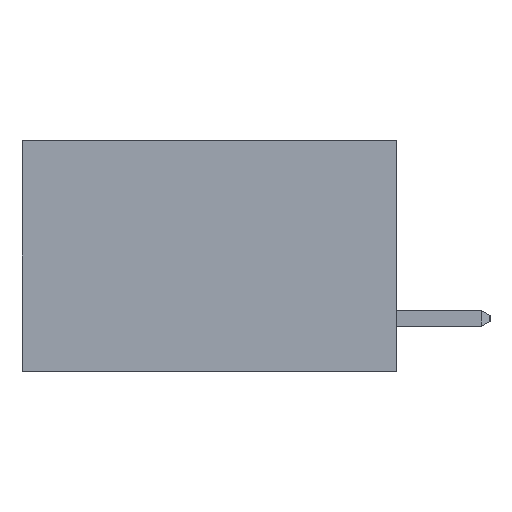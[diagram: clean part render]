
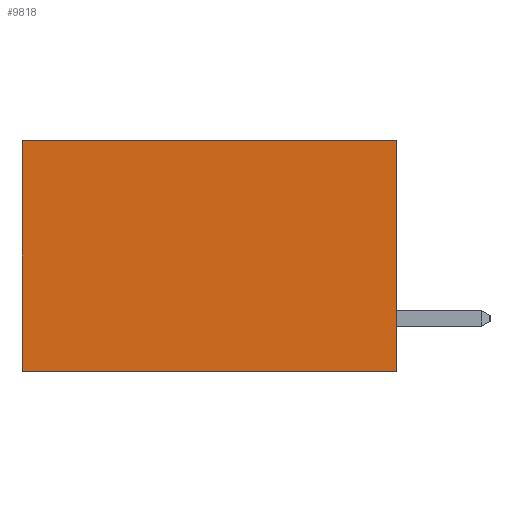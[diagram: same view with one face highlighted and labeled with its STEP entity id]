
A CAD part, left-side view. The second image highlights one B-rep face of the part: STEP entity #9818.
In plain terms, the highlighted planar face has unit normal (-1, 0, 0).
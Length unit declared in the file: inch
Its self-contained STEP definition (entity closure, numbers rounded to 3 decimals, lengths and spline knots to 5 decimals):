
#270 = CARTESIAN_POINT ( 'NONE',  ( 0.298, 0., 0. ) ) ;
#298 = LINE ( 'NONE', #11627, #12478 ) ;
#893 = VERTEX_POINT ( 'NONE', #12988 ) ;
#1684 = VERTEX_POINT ( 'NONE', #5864 ) ;
#2046 = LINE ( 'NONE', #10620, #7878 ) ;
#2406 = EDGE_LOOP ( 'NONE', ( #6444, #13858, #11704, #6688 ) ) ;
#2686 = DIRECTION ( 'NONE',  ( 0., 0., -1. ) ) ;
#3616 = CARTESIAN_POINT ( 'NONE',  ( 0.298, 0., -0.37 ) ) ;
#4255 = VERTEX_POINT ( 'NONE', #12004 ) ;
#4386 = VECTOR ( 'NONE', #2686, 39.37008 ) ;
#4755 = LINE ( 'NONE', #270, #4386 ) ;
#5110 = AXIS2_PLACEMENT_3D ( 'NONE', #6878, #6774, #6847 ) ;
#5672 = VERTEX_POINT ( 'NONE', #10574 ) ;
#5864 = CARTESIAN_POINT ( 'NONE',  ( 0.298, 0.6, 0. ) ) ;
#6444 = ORIENTED_EDGE ( 'NONE', *, *, #7869, .T. ) ;
#6688 = ORIENTED_EDGE ( 'NONE', *, *, #7137, .T. ) ;
#6774 = DIRECTION ( 'NONE',  ( 1., 0., 0. ) ) ;
#6847 = DIRECTION ( 'NONE',  ( 0., 0., -1. ) ) ;
#6878 = CARTESIAN_POINT ( 'NONE',  ( 0.298, 0., 0. ) ) ;
#7002 = PLANE ( 'NONE',  #5110 ) ;
#7032 = DIRECTION ( 'NONE',  ( 0., 1., 0. ) ) ;
#7040 = EDGE_CURVE ( 'NONE', #4255, #5672, #4755, .T. ) ;
#7137 = EDGE_CURVE ( 'NONE', #4255, #1684, #298, .T. ) ;
#7869 = EDGE_CURVE ( 'NONE', #1684, #893, #2046, .T. ) ;
#7878 = VECTOR ( 'NONE', #10051, 39.37008 ) ;
#8053 = EDGE_CURVE ( 'NONE', #5672, #893, #11589, .T. ) ;
#9304 = FACE_OUTER_BOUND ( 'NONE', #2406, .T. ) ;
#9818 = ADVANCED_FACE ( 'NONE', ( #9304 ), #7002, .F. ) ;
#10051 = DIRECTION ( 'NONE',  ( 0., 0., -1. ) ) ;
#10574 = CARTESIAN_POINT ( 'NONE',  ( 0.298, 0., -0.37 ) ) ;
#10620 = CARTESIAN_POINT ( 'NONE',  ( 0.298, 0.6, 0. ) ) ;
#11589 = LINE ( 'NONE', #3616, #12331 ) ;
#11627 = CARTESIAN_POINT ( 'NONE',  ( 0.298, 0., 0. ) ) ;
#11704 = ORIENTED_EDGE ( 'NONE', *, *, #7040, .F. ) ;
#12004 = CARTESIAN_POINT ( 'NONE',  ( 0.298, 0., 0. ) ) ;
#12331 = VECTOR ( 'NONE', #7032, 39.37008 ) ;
#12478 = VECTOR ( 'NONE', #15547, 39.37008 ) ;
#12988 = CARTESIAN_POINT ( 'NONE',  ( 0.298, 0.6, -0.37 ) ) ;
#13858 = ORIENTED_EDGE ( 'NONE', *, *, #8053, .F. ) ;
#15547 = DIRECTION ( 'NONE',  ( 0., 1., 0. ) ) ;
